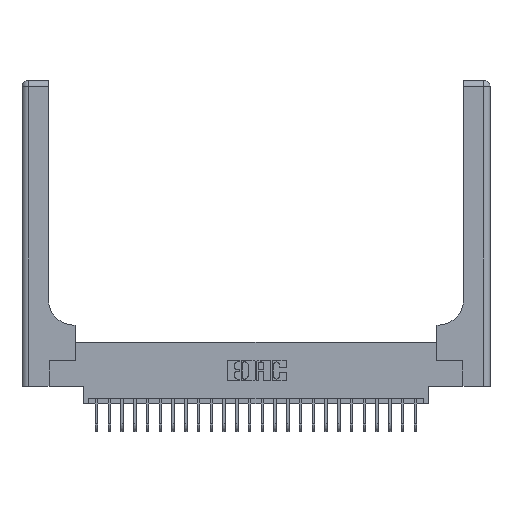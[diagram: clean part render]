
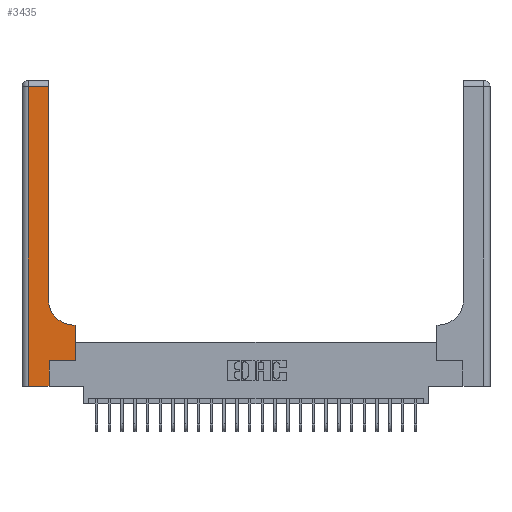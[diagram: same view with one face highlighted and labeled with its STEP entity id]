
A CAD part, top view. The second image highlights one B-rep face of the part: STEP entity #3435.
In plain terms, the highlighted planar face has unit normal (0, 0, 1).
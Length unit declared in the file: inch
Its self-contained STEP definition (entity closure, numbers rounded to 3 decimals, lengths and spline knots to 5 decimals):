
#450 = CARTESIAN_POINT ( 'NONE',  ( 0.528, 0.25, 0.37 ) ) ;
#705 = CARTESIAN_POINT ( 'NONE',  ( 0.26, 0.6, 0.37 ) ) ;
#1196 = CARTESIAN_POINT ( 'NONE',  ( 0.265, 0.25, 0.37 ) ) ;
#1206 = VECTOR ( 'NONE', #10578, 39.37008 ) ;
#1589 = CARTESIAN_POINT ( 'NONE',  ( 0.51, 0.85, 0.37 ) ) ;
#1672 = DIRECTION ( 'NONE',  ( 1., 0., 0. ) ) ;
#2431 = VERTEX_POINT ( 'NONE', #450 ) ;
#2564 = VERTEX_POINT ( 'NONE', #13382 ) ;
#3435 = ADVANCED_FACE ( 'NONE', ( #15600 ), #23179, .F. ) ;
#3908 = EDGE_CURVE ( 'NONE', #17402, #13200, #23870, .T. ) ;
#4499 = CARTESIAN_POINT ( 'NONE',  ( 0.06, 3., 0.37 ) ) ;
#5254 = ORIENTED_EDGE ( 'NONE', *, *, #10551, .T. ) ;
#5507 = VECTOR ( 'NONE', #11669, 39.37008 ) ;
#6083 = EDGE_LOOP ( 'NONE', ( #9331, #13754, #21861, #18651, #9026, #7751, #5254, #17462, #8844 ) ) ;
#6282 = CARTESIAN_POINT ( 'NONE',  ( 0.26, 0.85, 0.37 ) ) ;
#6329 = EDGE_CURVE ( 'NONE', #12133, #2564, #12007, .T. ) ;
#6960 = CARTESIAN_POINT ( 'NONE',  ( 0.265, 0., 0.37 ) ) ;
#7039 = LINE ( 'NONE', #10586, #19134 ) ;
#7751 = ORIENTED_EDGE ( 'NONE', *, *, #23081, .T. ) ;
#7788 = CARTESIAN_POINT ( 'NONE',  ( 0.51, 0.6, 0.37 ) ) ;
#8100 = DIRECTION ( 'NONE',  ( 0., 1., 0. ) ) ;
#8844 = ORIENTED_EDGE ( 'NONE', *, *, #10214, .T. ) ;
#9026 = ORIENTED_EDGE ( 'NONE', *, *, #3908, .T. ) ;
#9331 = ORIENTED_EDGE ( 'NONE', *, *, #6329, .T. ) ;
#10214 = EDGE_CURVE ( 'NONE', #13114, #12133, #16395, .T. ) ;
#10331 = CARTESIAN_POINT ( 'NONE',  ( 0.265, 0., 0.37 ) ) ;
#10551 = EDGE_CURVE ( 'NONE', #2431, #13755, #7039, .T. ) ;
#10578 = DIRECTION ( 'NONE',  ( 0., 1., 0. ) ) ;
#10586 = CARTESIAN_POINT ( 'NONE',  ( 0.528, 0.25, 0.37 ) ) ;
#10805 = EDGE_CURVE ( 'NONE', #21651, #17402, #20834, .T. ) ;
#11343 = DIRECTION ( 'NONE',  ( 1., 0., 0. ) ) ;
#11589 = DIRECTION ( 'NONE',  ( -1., 0., 0. ) ) ;
#11669 = DIRECTION ( 'NONE',  ( 1., 0., 0. ) ) ;
#11749 = EDGE_CURVE ( 'NONE', #13755, #13114, #13404, .T. ) ;
#11774 = CARTESIAN_POINT ( 'NONE',  ( 0.26, 3., 0.37 ) ) ;
#11834 = DIRECTION ( 'NONE',  ( -1., 0., 0. ) ) ;
#12007 = LINE ( 'NONE', #11774, #18481 ) ;
#12133 = VERTEX_POINT ( 'NONE', #6282 ) ;
#12887 = CARTESIAN_POINT ( 'NONE',  ( 0.265, 0.25, 0.37 ) ) ;
#13114 = VERTEX_POINT ( 'NONE', #7788 ) ;
#13200 = VERTEX_POINT ( 'NONE', #1196 ) ;
#13382 = CARTESIAN_POINT ( 'NONE',  ( 0.26, 2.94, 0.37 ) ) ;
#13404 = LINE ( 'NONE', #705, #17553 ) ;
#13648 = DIRECTION ( 'NONE',  ( 0., 0., -1. ) ) ;
#13754 = ORIENTED_EDGE ( 'NONE', *, *, #20624, .T. ) ;
#13755 = VERTEX_POINT ( 'NONE', #14461 ) ;
#13899 = VECTOR ( 'NONE', #18774, 39.37008 ) ;
#14043 = AXIS2_PLACEMENT_3D ( 'NONE', #1589, #18567, #11343 ) ;
#14461 = CARTESIAN_POINT ( 'NONE',  ( 0.528, 0.6, 0.37 ) ) ;
#14705 = VECTOR ( 'NONE', #19390, 39.37008 ) ;
#15600 = FACE_OUTER_BOUND ( 'NONE', #6083, .T. ) ;
#15668 = VERTEX_POINT ( 'NONE', #19076 ) ;
#16395 = CIRCLE ( 'NONE', #14043, 0.25 ) ;
#16691 = CARTESIAN_POINT ( 'NONE',  ( 0., 2.94, 0.37 ) ) ;
#16704 = VECTOR ( 'NONE', #1672, 39.37008 ) ;
#17402 = VERTEX_POINT ( 'NONE', #6960 ) ;
#17462 = ORIENTED_EDGE ( 'NONE', *, *, #11749, .T. ) ;
#17553 = VECTOR ( 'NONE', #11589, 39.37008 ) ;
#18365 = AXIS2_PLACEMENT_3D ( 'NONE', #21120, #13648, #11834 ) ;
#18402 = LINE ( 'NONE', #12887, #16704 ) ;
#18481 = VECTOR ( 'NONE', #8100, 39.37008 ) ;
#18567 = DIRECTION ( 'NONE',  ( 0., 0., -1. ) ) ;
#18651 = ORIENTED_EDGE ( 'NONE', *, *, #10805, .T. ) ;
#18774 = DIRECTION ( 'NONE',  ( -1., 0., 0. ) ) ;
#19076 = CARTESIAN_POINT ( 'NONE',  ( 0.06, 2.94, 0.37 ) ) ;
#19134 = VECTOR ( 'NONE', #19606, 39.37008 ) ;
#19390 = DIRECTION ( 'NONE',  ( 0., -1., 0. ) ) ;
#19502 = LINE ( 'NONE', #4499, #14705 ) ;
#19606 = DIRECTION ( 'NONE',  ( 0., 1., 0. ) ) ;
#20624 = EDGE_CURVE ( 'NONE', #2564, #15668, #22307, .T. ) ;
#20834 = LINE ( 'NONE', #22543, #5507 ) ;
#21120 = CARTESIAN_POINT ( 'NONE',  ( 0., 3., 0.37 ) ) ;
#21445 = EDGE_CURVE ( 'NONE', #15668, #21651, #19502, .T. ) ;
#21651 = VERTEX_POINT ( 'NONE', #24131 ) ;
#21861 = ORIENTED_EDGE ( 'NONE', *, *, #21445, .T. ) ;
#22307 = LINE ( 'NONE', #16691, #13899 ) ;
#22543 = CARTESIAN_POINT ( 'NONE',  ( 0., 0., 0.37 ) ) ;
#23081 = EDGE_CURVE ( 'NONE', #13200, #2431, #18402, .T. ) ;
#23179 = PLANE ( 'NONE',  #18365 ) ;
#23870 = LINE ( 'NONE', #10331, #1206 ) ;
#24131 = CARTESIAN_POINT ( 'NONE',  ( 0.06, 0., 0.37 ) ) ;
